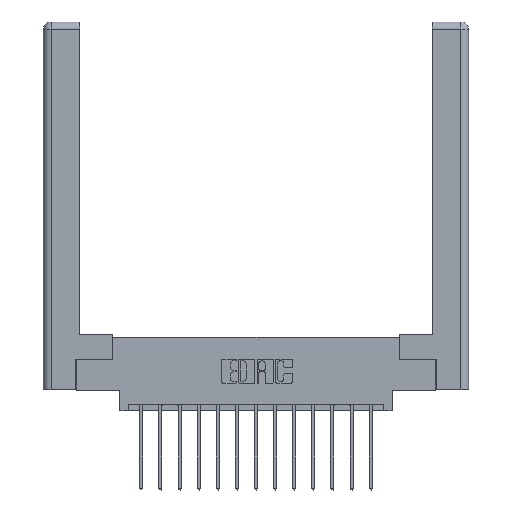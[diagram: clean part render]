
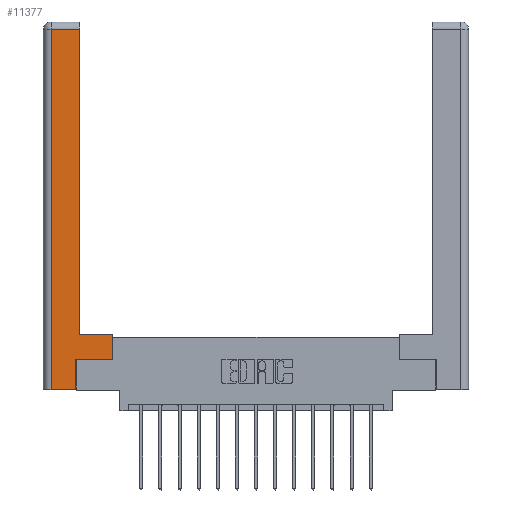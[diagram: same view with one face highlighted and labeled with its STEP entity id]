
A CAD part, top view. The second image highlights one B-rep face of the part: STEP entity #11377.
In plain terms, the highlighted planar face has unit normal (0, 0, 1).
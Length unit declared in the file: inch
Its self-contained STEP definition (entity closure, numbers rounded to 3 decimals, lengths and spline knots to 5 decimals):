
#199 = EDGE_CURVE ( 'NONE', #7515, #5483, #4386, .T. ) ;
#202 = DIRECTION ( 'NONE',  ( -1., 0., 0. ) ) ;
#494 = VERTEX_POINT ( 'NONE', #970 ) ;
#970 = CARTESIAN_POINT ( 'NONE',  ( 0.0615, 0., 0. ) ) ;
#1418 = CARTESIAN_POINT ( 'NONE',  ( 0.0615, 0., 0. ) ) ;
#1453 = CARTESIAN_POINT ( 'NONE',  ( 0.0615, 2.94, 0. ) ) ;
#1583 = CARTESIAN_POINT ( 'NONE',  ( 0.565, 0.245, 0. ) ) ;
#1776 = LINE ( 'NONE', #1418, #14650 ) ;
#1787 = VECTOR ( 'NONE', #3710, 39.37008 ) ;
#1903 = CARTESIAN_POINT ( 'NONE',  ( 0.565, 0.245, 0. ) ) ;
#2036 = DIRECTION ( 'NONE',  ( 1., 0., 0. ) ) ;
#2273 = VECTOR ( 'NONE', #6446, 39.37008 ) ;
#2520 = CARTESIAN_POINT ( 'NONE',  ( 0.565, 0.45, 0. ) ) ;
#3252 = LINE ( 'NONE', #11498, #2273 ) ;
#3710 = DIRECTION ( 'NONE',  ( 0., 1., 0. ) ) ;
#4243 = VERTEX_POINT ( 'NONE', #1583 ) ;
#4386 = LINE ( 'NONE', #10116, #1787 ) ;
#4483 = LINE ( 'NONE', #14921, #15376 ) ;
#4573 = ORIENTED_EDGE ( 'NONE', *, *, #15256, .T. ) ;
#4581 = ORIENTED_EDGE ( 'NONE', *, *, #13942, .T. ) ;
#4706 = EDGE_CURVE ( 'NONE', #494, #15318, #10196, .T. ) ;
#5131 = CARTESIAN_POINT ( 'NONE',  ( 0.265, 0., 0. ) ) ;
#5483 = VERTEX_POINT ( 'NONE', #12021 ) ;
#5854 = DIRECTION ( 'NONE',  ( -1., 0., 0. ) ) ;
#6113 = EDGE_CURVE ( 'NONE', #7913, #4243, #14313, .T. ) ;
#6446 = DIRECTION ( 'NONE',  ( 0., 1., 0. ) ) ;
#6615 = DIRECTION ( 'NONE',  ( 0., -1., 0. ) ) ;
#6652 = VECTOR ( 'NONE', #8515, 39.37008 ) ;
#7010 = AXIS2_PLACEMENT_3D ( 'NONE', #13770, #11238, #5854 ) ;
#7056 = CARTESIAN_POINT ( 'NONE',  ( 0.0615, 2.94, 0. ) ) ;
#7284 = DIRECTION ( 'NONE',  ( -1., 0., 0. ) ) ;
#7299 = EDGE_LOOP ( 'NONE', ( #7524, #4581, #15365, #13300, #4573, #14444, #13863, #13021 ) ) ;
#7515 = VERTEX_POINT ( 'NONE', #9189 ) ;
#7524 = ORIENTED_EDGE ( 'NONE', *, *, #199, .T. ) ;
#7568 = VECTOR ( 'NONE', #202, 39.37008 ) ;
#7913 = VERTEX_POINT ( 'NONE', #12662 ) ;
#7985 = EDGE_CURVE ( 'NONE', #15555, #494, #1776, .T. ) ;
#8047 = LINE ( 'NONE', #16121, #6652 ) ;
#8154 = LINE ( 'NONE', #1453, #7568 ) ;
#8329 = PLANE ( 'NONE',  #7010 ) ;
#8515 = DIRECTION ( 'NONE',  ( 0., 1., 0. ) ) ;
#8720 = VECTOR ( 'NONE', #13492, 39.37008 ) ;
#9189 = CARTESIAN_POINT ( 'NONE',  ( 0.295, 0.45, 0. ) ) ;
#10116 = CARTESIAN_POINT ( 'NONE',  ( 0.295, 3., 0. ) ) ;
#10196 = LINE ( 'NONE', #12220, #10763 ) ;
#10763 = VECTOR ( 'NONE', #2036, 39.37008 ) ;
#10830 = VERTEX_POINT ( 'NONE', #2520 ) ;
#11238 = DIRECTION ( 'NONE',  ( 0., 0., -1. ) ) ;
#11377 = ADVANCED_FACE ( 'NONE', ( #15483 ), #8329, .F. ) ;
#11498 = CARTESIAN_POINT ( 'NONE',  ( 0.265, 0.245, 0. ) ) ;
#12021 = CARTESIAN_POINT ( 'NONE',  ( 0.295, 2.94, 0. ) ) ;
#12220 = CARTESIAN_POINT ( 'NONE',  ( 0.265, 0., 0. ) ) ;
#12662 = CARTESIAN_POINT ( 'NONE',  ( 0.265, 0.245, 0. ) ) ;
#13021 = ORIENTED_EDGE ( 'NONE', *, *, #14559, .T. ) ;
#13300 = ORIENTED_EDGE ( 'NONE', *, *, #4706, .T. ) ;
#13492 = DIRECTION ( 'NONE',  ( 1., 0., 0. ) ) ;
#13770 = CARTESIAN_POINT ( 'NONE',  ( 0., 0., 0. ) ) ;
#13863 = ORIENTED_EDGE ( 'NONE', *, *, #16387, .T. ) ;
#13942 = EDGE_CURVE ( 'NONE', #5483, #15555, #8154, .T. ) ;
#14313 = LINE ( 'NONE', #1903, #8720 ) ;
#14444 = ORIENTED_EDGE ( 'NONE', *, *, #6113, .T. ) ;
#14559 = EDGE_CURVE ( 'NONE', #10830, #7515, #4483, .T. ) ;
#14650 = VECTOR ( 'NONE', #6615, 39.37008 ) ;
#14921 = CARTESIAN_POINT ( 'NONE',  ( 0.295, 0.45, 0. ) ) ;
#15256 = EDGE_CURVE ( 'NONE', #15318, #7913, #3252, .T. ) ;
#15318 = VERTEX_POINT ( 'NONE', #5131 ) ;
#15365 = ORIENTED_EDGE ( 'NONE', *, *, #7985, .T. ) ;
#15376 = VECTOR ( 'NONE', #7284, 39.37008 ) ;
#15483 = FACE_OUTER_BOUND ( 'NONE', #7299, .T. ) ;
#15555 = VERTEX_POINT ( 'NONE', #7056 ) ;
#16121 = CARTESIAN_POINT ( 'NONE',  ( 0.565, 0.45, 0. ) ) ;
#16387 = EDGE_CURVE ( 'NONE', #4243, #10830, #8047, .T. ) ;
